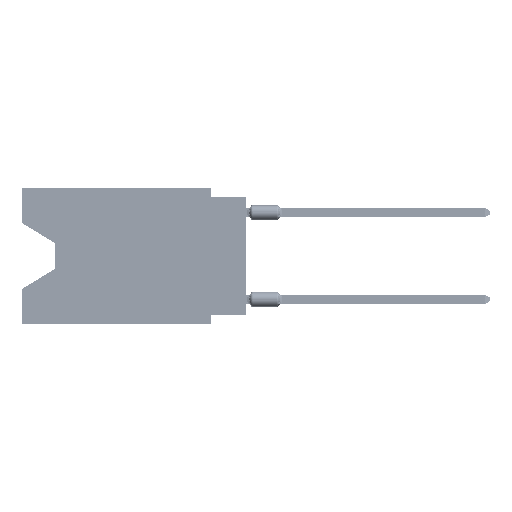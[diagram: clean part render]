
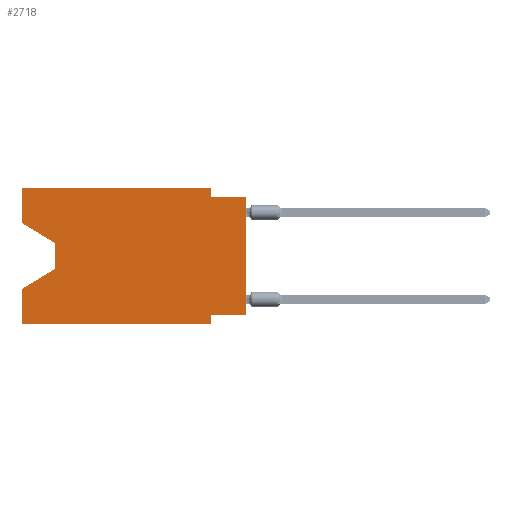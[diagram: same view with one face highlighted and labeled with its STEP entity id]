
A CAD part, left-side view. The second image highlights one B-rep face of the part: STEP entity #2718.
In plain terms, the highlighted planar face has unit normal (-1, 0, 0).
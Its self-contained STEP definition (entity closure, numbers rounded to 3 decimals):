
#264 = EDGE_CURVE ( 'NONE', #26910, #44617, #30255, .T. ) ;
#405 = LINE ( 'NONE', #24749, #6970 ) ;
#1596 = DIRECTION ( 'NONE',  ( 0., 0., -1. ) ) ;
#2212 = ORIENTED_EDGE ( 'NONE', *, *, #60659, .T. ) ;
#2718 = ADVANCED_FACE ( 'NONE', ( #66558 ), #29201, .F. ) ;
#2942 = EDGE_LOOP ( 'NONE', ( #2212, #24603, #76442, #32023, #25801, #44559, #43581, #45313, #70905, #70341, #76307, #33918 ) ) ;
#4326 = VECTOR ( 'NONE', #35551, 1000. ) ;
#4910 = DIRECTION ( 'NONE',  ( 0., 0., 1. ) ) ;
#5322 = VECTOR ( 'NONE', #19351, 1000. ) ;
#6071 = EDGE_CURVE ( 'NONE', #70608, #52747, #33789, .T. ) ;
#6970 = VECTOR ( 'NONE', #1596, 1000. ) ;
#10540 = DIRECTION ( 'NONE',  ( 1., 0., 0. ) ) ;
#10745 = VERTEX_POINT ( 'NONE', #61129 ) ;
#10884 = CARTESIAN_POINT ( 'NONE',  ( 0., 0., -0.635 ) ) ;
#14533 = CARTESIAN_POINT ( 'NONE',  ( 0., 2.54, -9.906 ) ) ;
#16693 = CARTESIAN_POINT ( 'NONE',  ( 0., 16.383, 0. ) ) ;
#16802 = DIRECTION ( 'NONE',  ( 0., -1., 0. ) ) ;
#19351 = DIRECTION ( 'NONE',  ( 0., -0.855, -0.519 ) ) ;
#23005 = VERTEX_POINT ( 'NONE', #44974 ) ;
#24254 = DIRECTION ( 'NONE',  ( 0., 1., 0. ) ) ;
#24603 = ORIENTED_EDGE ( 'NONE', *, *, #264, .T. ) ;
#24628 = VECTOR ( 'NONE', #30786, 1000. ) ;
#24749 = CARTESIAN_POINT ( 'NONE',  ( 0., 2.54, 0. ) ) ;
#25002 = VECTOR ( 'NONE', #4910, 1000. ) ;
#25443 = LINE ( 'NONE', #50198, #5322 ) ;
#25801 = ORIENTED_EDGE ( 'NONE', *, *, #48720, .T. ) ;
#26910 = VERTEX_POINT ( 'NONE', #79468 ) ;
#28284 = CARTESIAN_POINT ( 'NONE',  ( 0., 13.97, -5.893 ) ) ;
#29201 = PLANE ( 'NONE',  #78523 ) ;
#30255 = LINE ( 'NONE', #42412, #4326 ) ;
#30626 = CARTESIAN_POINT ( 'NONE',  ( 0., 16.383, 0. ) ) ;
#30786 = DIRECTION ( 'NONE',  ( 0., 0., 1. ) ) ;
#32023 = ORIENTED_EDGE ( 'NONE', *, *, #62729, .F. ) ;
#33195 = LINE ( 'NONE', #28284, #70326 ) ;
#33789 = LINE ( 'NONE', #51650, #80142 ) ;
#33918 = ORIENTED_EDGE ( 'NONE', *, *, #62666, .F. ) ;
#35551 = DIRECTION ( 'NONE',  ( 0., 0., -1. ) ) ;
#35765 = CARTESIAN_POINT ( 'NONE',  ( 0., 16.383, 0. ) ) ;
#37346 = CARTESIAN_POINT ( 'NONE',  ( 0., 0., -9.271 ) ) ;
#37788 = CARTESIAN_POINT ( 'NONE',  ( 0., 2.54, 0. ) ) ;
#40686 = VECTOR ( 'NONE', #24254, 1000. ) ;
#40974 = DIRECTION ( 'NONE',  ( 0., 0., -1. ) ) ;
#41705 = CARTESIAN_POINT ( 'NONE',  ( 0., 2.54, -9.906 ) ) ;
#42412 = CARTESIAN_POINT ( 'NONE',  ( 0., 13.97, -4.013 ) ) ;
#42420 = EDGE_CURVE ( 'NONE', #44617, #23005, #33195, .T. ) ;
#43128 = CARTESIAN_POINT ( 'NONE',  ( 0., 16.383, -9.906 ) ) ;
#43581 = ORIENTED_EDGE ( 'NONE', *, *, #44295, .F. ) ;
#43914 = EDGE_CURVE ( 'NONE', #52747, #67587, #405, .T. ) ;
#44295 = EDGE_CURVE ( 'NONE', #48028, #73160, #55892, .T. ) ;
#44559 = ORIENTED_EDGE ( 'NONE', *, *, #70223, .F. ) ;
#44617 = VERTEX_POINT ( 'NONE', #71729 ) ;
#44974 = CARTESIAN_POINT ( 'NONE',  ( 0., 16.383, -7.36 ) ) ;
#45313 = ORIENTED_EDGE ( 'NONE', *, *, #60431, .T. ) ;
#47799 = LINE ( 'NONE', #41705, #50762 ) ;
#48028 = VERTEX_POINT ( 'NONE', #37346 ) ;
#48333 = LINE ( 'NONE', #16693, #49634 ) ;
#48720 = EDGE_CURVE ( 'NONE', #65719, #64664, #72439, .T. ) ;
#49634 = VECTOR ( 'NONE', #73534, 1000. ) ;
#50198 = CARTESIAN_POINT ( 'NONE',  ( 0., 16.383, -2.546 ) ) ;
#50762 = VECTOR ( 'NONE', #55081, 1000. ) ;
#51650 = CARTESIAN_POINT ( 'NONE',  ( 0., 16.383, 0. ) ) ;
#52053 = DIRECTION ( 'NONE',  ( 0., -1., 0. ) ) ;
#52747 = VERTEX_POINT ( 'NONE', #37788 ) ;
#53543 = CARTESIAN_POINT ( 'NONE',  ( 0., 16.383, -9.906 ) ) ;
#54682 = LINE ( 'NONE', #10884, #77998 ) ;
#55081 = DIRECTION ( 'NONE',  ( 0., 0., -1. ) ) ;
#55100 = CARTESIAN_POINT ( 'NONE',  ( 0., 0., -9.271 ) ) ;
#55892 = LINE ( 'NONE', #55100, #40686 ) ;
#60126 = LINE ( 'NONE', #35765, #25002 ) ;
#60431 = EDGE_CURVE ( 'NONE', #48028, #69467, #67745, .T. ) ;
#60659 = EDGE_CURVE ( 'NONE', #10745, #26910, #25443, .T. ) ;
#61129 = CARTESIAN_POINT ( 'NONE',  ( 0., 16.383, -2.546 ) ) ;
#61647 = CARTESIAN_POINT ( 'NONE',  ( 0., 0., 0. ) ) ;
#62666 = EDGE_CURVE ( 'NONE', #10745, #70608, #48333, .T. ) ;
#62729 = EDGE_CURVE ( 'NONE', #65719, #23005, #60126, .T. ) ;
#64212 = CARTESIAN_POINT ( 'NONE',  ( 0., 0., -0.635 ) ) ;
#64664 = VERTEX_POINT ( 'NONE', #14533 ) ;
#65719 = VERTEX_POINT ( 'NONE', #53543 ) ;
#66460 = CARTESIAN_POINT ( 'NONE',  ( 0., 2.54, -0.635 ) ) ;
#66558 = FACE_OUTER_BOUND ( 'NONE', #2942, .T. ) ;
#67587 = VERTEX_POINT ( 'NONE', #66460 ) ;
#67745 = LINE ( 'NONE', #61647, #24628 ) ;
#69467 = VERTEX_POINT ( 'NONE', #64212 ) ;
#70143 = DIRECTION ( 'NONE',  ( 0., 0.855, -0.519 ) ) ;
#70223 = EDGE_CURVE ( 'NONE', #73160, #64664, #47799, .T. ) ;
#70224 = EDGE_CURVE ( 'NONE', #67587, #69467, #54682, .T. ) ;
#70326 = VECTOR ( 'NONE', #70143, 1000. ) ;
#70341 = ORIENTED_EDGE ( 'NONE', *, *, #43914, .F. ) ;
#70608 = VERTEX_POINT ( 'NONE', #30626 ) ;
#70905 = ORIENTED_EDGE ( 'NONE', *, *, #70224, .F. ) ;
#71729 = CARTESIAN_POINT ( 'NONE',  ( 0., 13.97, -5.893 ) ) ;
#72120 = VECTOR ( 'NONE', #16802, 1000. ) ;
#72439 = LINE ( 'NONE', #43128, #72120 ) ;
#72658 = CARTESIAN_POINT ( 'NONE',  ( 0., 16.383, 0. ) ) ;
#73160 = VERTEX_POINT ( 'NONE', #74919 ) ;
#73534 = DIRECTION ( 'NONE',  ( 0., 0., 1. ) ) ;
#74919 = CARTESIAN_POINT ( 'NONE',  ( 0., 2.54, -9.271 ) ) ;
#76307 = ORIENTED_EDGE ( 'NONE', *, *, #6071, .F. ) ;
#76442 = ORIENTED_EDGE ( 'NONE', *, *, #42420, .T. ) ;
#77998 = VECTOR ( 'NONE', #79084, 1000. ) ;
#78523 = AXIS2_PLACEMENT_3D ( 'NONE', #72658, #10540, #40974 ) ;
#79084 = DIRECTION ( 'NONE',  ( 0., -1., 0. ) ) ;
#79468 = CARTESIAN_POINT ( 'NONE',  ( 0., 13.97, -4.013 ) ) ;
#80142 = VECTOR ( 'NONE', #52053, 1000. ) ;
